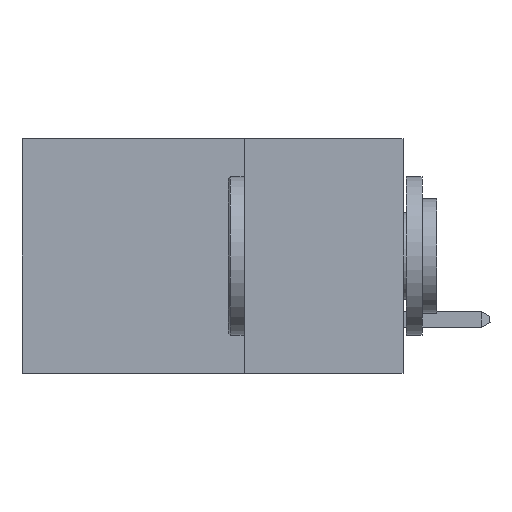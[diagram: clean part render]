
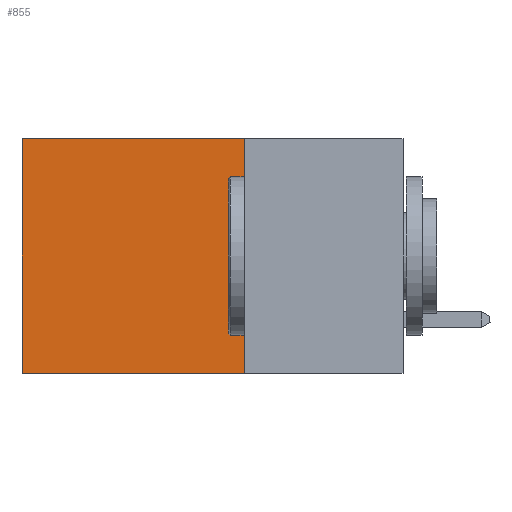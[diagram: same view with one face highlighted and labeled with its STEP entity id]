
A CAD part, left-side view. The second image highlights one B-rep face of the part: STEP entity #855.
In plain terms, the highlighted planar face has unit normal (-1, 0, 0).
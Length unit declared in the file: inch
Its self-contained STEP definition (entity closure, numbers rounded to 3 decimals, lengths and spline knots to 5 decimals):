
#615 = CARTESIAN_POINT ( 'NONE',  ( 0.2875, 0.25, 0. ) ) ;
#855 = ADVANCED_FACE ( 'NONE', ( #9973 ), #23220, .F. ) ;
#1332 = ORIENTED_EDGE ( 'NONE', *, *, #17916, .T. ) ;
#2309 = VERTEX_POINT ( 'NONE', #17214 ) ;
#2470 = DIRECTION ( 'NONE',  ( 0., 0., -1. ) ) ;
#2632 = ORIENTED_EDGE ( 'NONE', *, *, #12752, .F. ) ;
#4352 = VECTOR ( 'NONE', #7026, 39.37008 ) ;
#5114 = ORIENTED_EDGE ( 'NONE', *, *, #19551, .F. ) ;
#6336 = VERTEX_POINT ( 'NONE', #615 ) ;
#7026 = DIRECTION ( 'NONE',  ( 0., 0., -1. ) ) ;
#9242 = LINE ( 'NONE', #17801, #4352 ) ;
#9973 = FACE_OUTER_BOUND ( 'NONE', #18922, .T. ) ;
#10371 = CARTESIAN_POINT ( 'NONE',  ( 0.2875, 0.6, 0. ) ) ;
#11601 = LINE ( 'NONE', #16183, #20620 ) ;
#12752 = EDGE_CURVE ( 'NONE', #16197, #2309, #23278, .T. ) ;
#12906 = EDGE_CURVE ( 'NONE', #6336, #14706, #19887, .T. ) ;
#13679 = CARTESIAN_POINT ( 'NONE',  ( 0.2875, 0.25, -0.37 ) ) ;
#13709 = VECTOR ( 'NONE', #17288, 39.37008 ) ;
#14706 = VERTEX_POINT ( 'NONE', #10371 ) ;
#15134 = VECTOR ( 'NONE', #19485, 39.37008 ) ;
#16090 = CARTESIAN_POINT ( 'NONE',  ( 0.2875, 0.25, -0.37 ) ) ;
#16183 = CARTESIAN_POINT ( 'NONE',  ( 0.2875, 0.25, 0. ) ) ;
#16197 = VERTEX_POINT ( 'NONE', #16090 ) ;
#17214 = CARTESIAN_POINT ( 'NONE',  ( 0.2875, 0.6, -0.37 ) ) ;
#17288 = DIRECTION ( 'NONE',  ( 0., 1., 0. ) ) ;
#17801 = CARTESIAN_POINT ( 'NONE',  ( 0.2875, 0.6, 0. ) ) ;
#17916 = EDGE_CURVE ( 'NONE', #14706, #2309, #9242, .T. ) ;
#17959 = DIRECTION ( 'NONE',  ( 0., 0., -1. ) ) ;
#17969 = ORIENTED_EDGE ( 'NONE', *, *, #12906, .T. ) ;
#18922 = EDGE_LOOP ( 'NONE', ( #1332, #2632, #5114, #17969 ) ) ;
#19485 = DIRECTION ( 'NONE',  ( 0., 1., 0. ) ) ;
#19493 = DIRECTION ( 'NONE',  ( 1., 0., 0. ) ) ;
#19551 = EDGE_CURVE ( 'NONE', #6336, #16197, #11601, .T. ) ;
#19887 = LINE ( 'NONE', #21244, #15134 ) ;
#20620 = VECTOR ( 'NONE', #17959, 39.37008 ) ;
#20698 = AXIS2_PLACEMENT_3D ( 'NONE', #22090, #19493, #2470 ) ;
#21244 = CARTESIAN_POINT ( 'NONE',  ( 0.2875, 0.25, 0. ) ) ;
#22090 = CARTESIAN_POINT ( 'NONE',  ( 0.2875, 0.25, 0. ) ) ;
#23220 = PLANE ( 'NONE',  #20698 ) ;
#23278 = LINE ( 'NONE', #13679, #13709 ) ;
